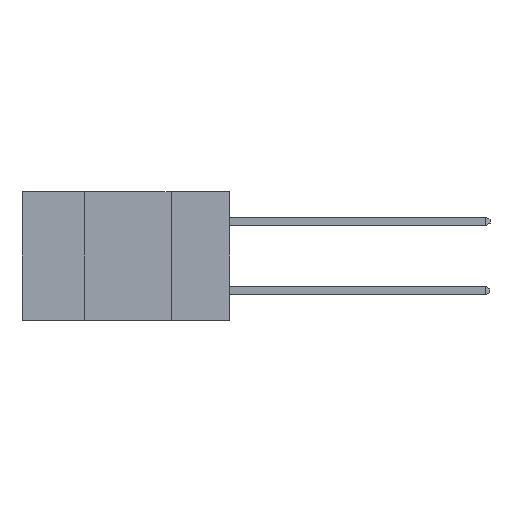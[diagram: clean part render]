
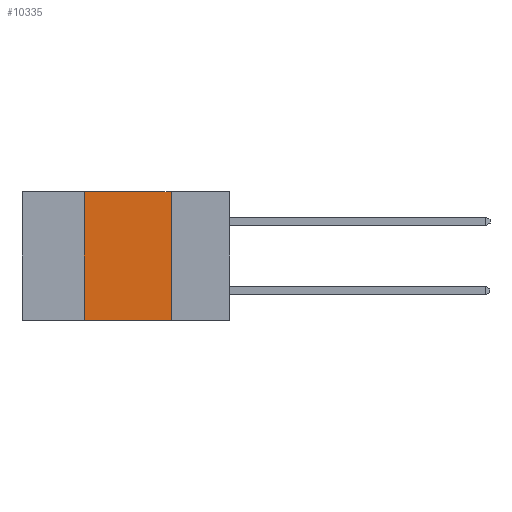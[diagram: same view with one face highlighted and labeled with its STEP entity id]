
A CAD part, left-side view. The second image highlights one B-rep face of the part: STEP entity #10335.
In plain terms, the highlighted planar face has unit normal (-1, 0, 0).
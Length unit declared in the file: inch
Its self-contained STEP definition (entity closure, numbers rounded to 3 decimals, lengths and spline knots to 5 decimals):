
#138 = CARTESIAN_POINT ( 'NONE',  ( 0., 0.42, 0. ) ) ;
#605 = DIRECTION ( 'NONE',  ( 1., 0., 0. ) ) ;
#952 = DIRECTION ( 'NONE',  ( 0., -1., 0. ) ) ;
#1234 = CARTESIAN_POINT ( 'NONE',  ( 0., 0.17, 0. ) ) ;
#1617 = CARTESIAN_POINT ( 'NONE',  ( 0., 0.42, 0. ) ) ;
#2019 = ORIENTED_EDGE ( 'NONE', *, *, #7744, .F. ) ;
#2758 = EDGE_CURVE ( 'NONE', #4709, #3853, #8072, .T. ) ;
#2988 = AXIS2_PLACEMENT_3D ( 'NONE', #9158, #605, #8162 ) ;
#3060 = VERTEX_POINT ( 'NONE', #1234 ) ;
#3434 = DIRECTION ( 'NONE',  ( 0., -1., 0. ) ) ;
#3540 = LINE ( 'NONE', #3901, #8998 ) ;
#3853 = VERTEX_POINT ( 'NONE', #6511 ) ;
#3901 = CARTESIAN_POINT ( 'NONE',  ( 0., 0.17, 0. ) ) ;
#4076 = LINE ( 'NONE', #1617, #7015 ) ;
#4709 = VERTEX_POINT ( 'NONE', #13571 ) ;
#5187 = VECTOR ( 'NONE', #952, 39.37008 ) ;
#5991 = PLANE ( 'NONE',  #2988 ) ;
#6320 = LINE ( 'NONE', #11001, #8841 ) ;
#6511 = CARTESIAN_POINT ( 'NONE',  ( 0., 0.17, -0.37 ) ) ;
#7015 = VECTOR ( 'NONE', #13390, 39.37008 ) ;
#7248 = CARTESIAN_POINT ( 'NONE',  ( 0., 0.6, -0.37 ) ) ;
#7744 = EDGE_CURVE ( 'NONE', #3060, #3853, #3540, .T. ) ;
#8072 = LINE ( 'NONE', #7248, #5187 ) ;
#8162 = DIRECTION ( 'NONE',  ( 0., 0., -1. ) ) ;
#8477 = ORIENTED_EDGE ( 'NONE', *, *, #2758, .T. ) ;
#8786 = VERTEX_POINT ( 'NONE', #138 ) ;
#8841 = VECTOR ( 'NONE', #3434, 39.37008 ) ;
#8998 = VECTOR ( 'NONE', #11395, 39.37008 ) ;
#9158 = CARTESIAN_POINT ( 'NONE',  ( 0., 0.6, 0. ) ) ;
#9925 = FACE_OUTER_BOUND ( 'NONE', #11076, .T. ) ;
#10335 = ADVANCED_FACE ( 'NONE', ( #9925 ), #5991, .F. ) ;
#11001 = CARTESIAN_POINT ( 'NONE',  ( 0., 0.6, 0. ) ) ;
#11076 = EDGE_LOOP ( 'NONE', ( #2019, #13781, #13451, #8477 ) ) ;
#11395 = DIRECTION ( 'NONE',  ( 0., 0., -1. ) ) ;
#12430 = EDGE_CURVE ( 'NONE', #4709, #8786, #4076, .T. ) ;
#12953 = EDGE_CURVE ( 'NONE', #8786, #3060, #6320, .T. ) ;
#13390 = DIRECTION ( 'NONE',  ( 0., 0., 1. ) ) ;
#13451 = ORIENTED_EDGE ( 'NONE', *, *, #12430, .F. ) ;
#13571 = CARTESIAN_POINT ( 'NONE',  ( 0., 0.42, -0.37 ) ) ;
#13781 = ORIENTED_EDGE ( 'NONE', *, *, #12953, .F. ) ;
